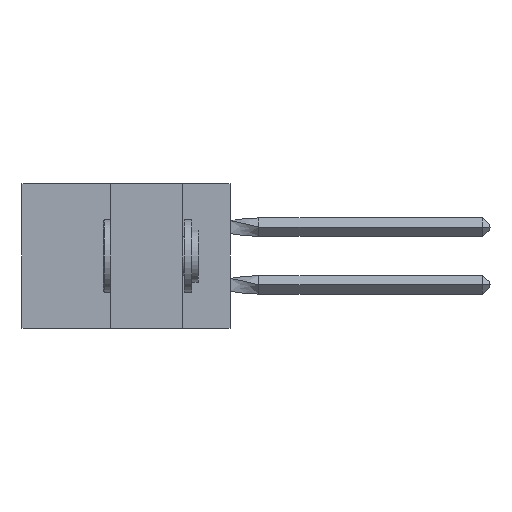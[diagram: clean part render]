
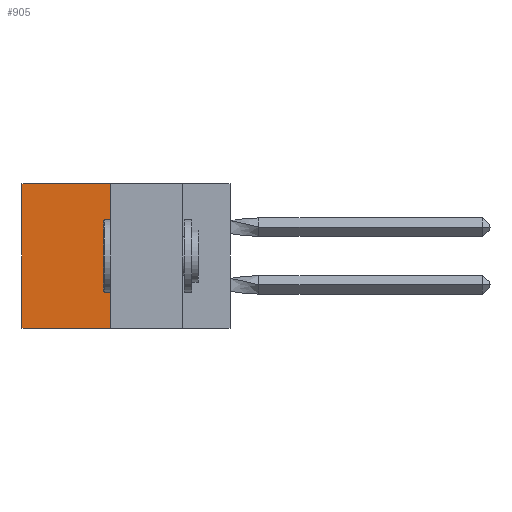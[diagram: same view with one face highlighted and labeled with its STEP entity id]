
A CAD part, left-side view. The second image highlights one B-rep face of the part: STEP entity #905.
In plain terms, the highlighted planar face has unit normal (-1, 0, 0).
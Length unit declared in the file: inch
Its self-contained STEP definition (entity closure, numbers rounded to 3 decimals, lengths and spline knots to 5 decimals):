
#208 = VERTEX_POINT ( 'NONE', #1486 ) ;
#479 = CARTESIAN_POINT ( 'NONE',  ( 0.305, 0.413, -0.5 ) ) ;
#905 = ADVANCED_FACE ( 'NONE', ( #20701 ), #20615, .F. ) ;
#1469 = EDGE_CURVE ( 'NONE', #7817, #4878, #7034, .T. ) ;
#1473 = EDGE_CURVE ( 'NONE', #11232, #4878, #20948, .T. ) ;
#1486 = CARTESIAN_POINT ( 'NONE',  ( 0.305, 0.413, 0. ) ) ;
#2755 = LINE ( 'NONE', #6787, #12996 ) ;
#4878 = VERTEX_POINT ( 'NONE', #18859 ) ;
#6754 = CARTESIAN_POINT ( 'NONE',  ( 0.305, 0.413, -0.5 ) ) ;
#6787 = CARTESIAN_POINT ( 'NONE',  ( 0.305, 0.413, 0. ) ) ;
#7034 = LINE ( 'NONE', #6754, #15819 ) ;
#7239 = CARTESIAN_POINT ( 'NONE',  ( 0.305, 0.413, -0.5 ) ) ;
#7257 = EDGE_CURVE ( 'NONE', #208, #7817, #14010, .T. ) ;
#7817 = VERTEX_POINT ( 'NONE', #479 ) ;
#9522 = DIRECTION ( 'NONE',  ( 0., 0., -1. ) ) ;
#9681 = CARTESIAN_POINT ( 'NONE',  ( 0.305, 0.413, -0.5 ) ) ;
#10292 = DIRECTION ( 'NONE',  ( 0., 0., -1. ) ) ;
#10707 = DIRECTION ( 'NONE',  ( 0., 0., -1. ) ) ;
#11232 = VERTEX_POINT ( 'NONE', #11917 ) ;
#11917 = CARTESIAN_POINT ( 'NONE',  ( 0.305, 0.72, 0. ) ) ;
#12134 = DIRECTION ( 'NONE',  ( 0., 1., 0. ) ) ;
#12433 = CARTESIAN_POINT ( 'NONE',  ( 0.305, 0.72, -0.5 ) ) ;
#12996 = VECTOR ( 'NONE', #23052, 39.37008 ) ;
#14010 = LINE ( 'NONE', #7239, #16568 ) ;
#14165 = AXIS2_PLACEMENT_3D ( 'NONE', #9681, #20375, #9522 ) ;
#14285 = ORIENTED_EDGE ( 'NONE', *, *, #1469, .F. ) ;
#15819 = VECTOR ( 'NONE', #12134, 39.37008 ) ;
#16568 = VECTOR ( 'NONE', #10707, 39.37008 ) ;
#17157 = EDGE_CURVE ( 'NONE', #208, #11232, #2755, .T. ) ;
#18859 = CARTESIAN_POINT ( 'NONE',  ( 0.305, 0.72, -0.5 ) ) ;
#19985 = EDGE_LOOP ( 'NONE', ( #21355, #14285, #22010, #23055 ) ) ;
#20375 = DIRECTION ( 'NONE',  ( 1., 0., 0. ) ) ;
#20615 = PLANE ( 'NONE',  #14165 ) ;
#20701 = FACE_OUTER_BOUND ( 'NONE', #19985, .T. ) ;
#20948 = LINE ( 'NONE', #12433, #21787 ) ;
#21355 = ORIENTED_EDGE ( 'NONE', *, *, #1473, .T. ) ;
#21787 = VECTOR ( 'NONE', #10292, 39.37008 ) ;
#22010 = ORIENTED_EDGE ( 'NONE', *, *, #7257, .F. ) ;
#23052 = DIRECTION ( 'NONE',  ( 0., 1., 0. ) ) ;
#23055 = ORIENTED_EDGE ( 'NONE', *, *, #17157, .T. ) ;
